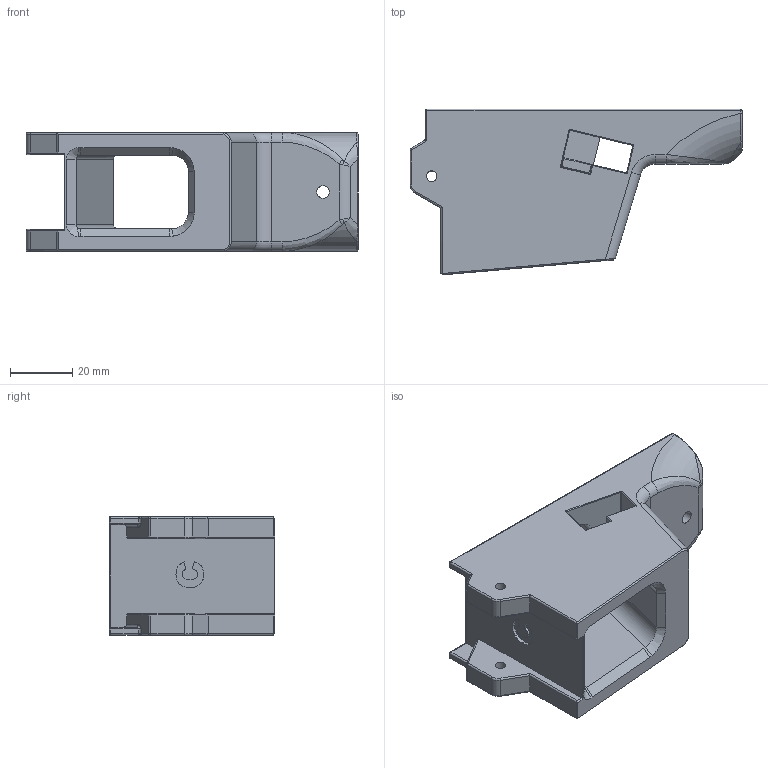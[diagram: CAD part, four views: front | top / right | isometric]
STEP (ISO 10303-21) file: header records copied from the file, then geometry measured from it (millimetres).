
FILE_DESCRIPTION(/* description */ (''),/* implementation_level */ '2;1');
FILE_NAME(/* author */ (''),/* organization */ (''),/* preprocessor_version */ 'ST-DEVELOPER v15.2',/* originating_system */ 'Autodesk Translator Framework v2.0.0.5431',/* authorisation */ '');
FILE_SCHEMA (('AUTOMOTIVE_DESIGN { 1 0 10303 214 3 1 1 }'));
Length unit declared in the file: centimetre
Products named in the file (1): MOD9 QUICK PRINT MAGWELL
Bounding box: 106.51 x 53.17 x 38 mm (x, y, z)
Volume: 87454.8 mm3; surface area: 25139.6 mm2
Topology: 1 solids, 1 shells, 291 faces, 726 edges, 432 vertices
Faces by surface type: bspline 94, plane 92, cylinder 78, torus 11, cone 10, sphere 6
Full cylindrical faces by diameter (mm): 1.5 x1, 3.4 x2, 4 x2
Entity records: 10313 total; most frequent: CARTESIAN_POINT 3924, ORIENTED_EDGE 1426, DIRECTION 1124, EDGE_CURVE 713, VERTEX_POINT 431, LINE 392, VECTOR 392, AXIS2_PLACEMENT_3D 366
